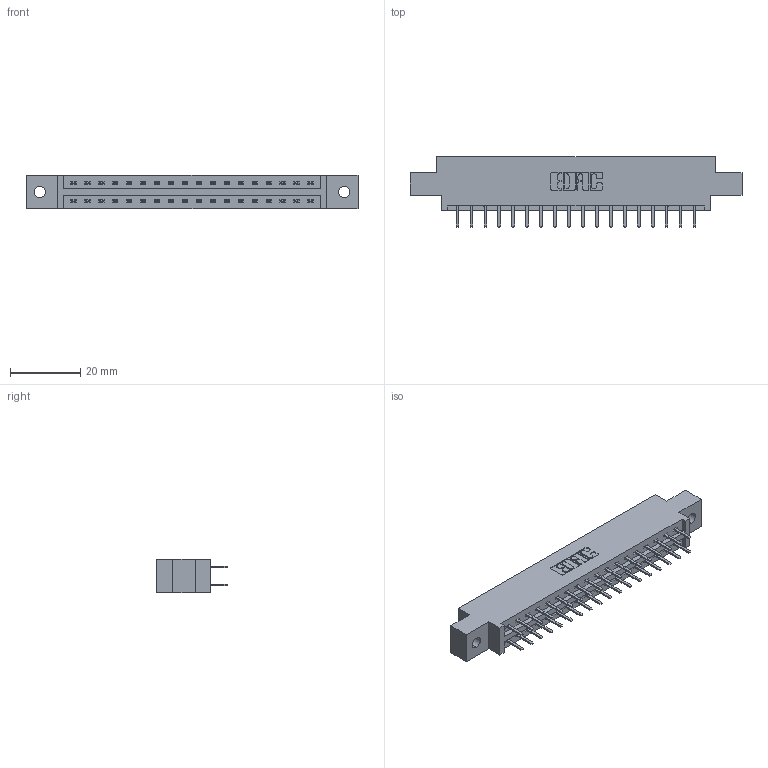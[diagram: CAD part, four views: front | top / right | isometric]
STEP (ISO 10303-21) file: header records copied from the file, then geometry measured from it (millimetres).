
FILE_DESCRIPTION (( 'STEP AP203' ), '1' );
FILE_NAME ('387-036-520-802.STEP', '2019-10-17T18:40:45', ( '' ), ( '' ), 'SwSTEP 2.0', 'SolidWorks 2016', '' );
FILE_SCHEMA (( 'CONFIG_CONTROL_DESIGN' ));
Length unit declared in the file: inch
Products named in the file (3): 345-292-001_345-293-120; 387-036-520-802; 337 Part_0.170 Offset - 0.128 Dia
Assembly tree (37 placements, depth 2):
  387-036-520-802
    337 Part_0.170 Offset - 0.128 Dia
    345-292-001_345-293-120  x36
Bounding box: 94.34 x 20.02 x 9.4 mm (x, y, z)
Volume: 9452.4 mm3; surface area: 10242.8 mm2
Topology: 37 solids, 37 shells, 2206 faces, 6407 edges, 4174 vertices
Faces by surface type: plane 1514, cylinder 692
Entity records: 17309 total; most frequent: CARTESIAN_POINT 2950, ORIENTED_EDGE 2874, DIRECTION 2541, EDGE_CURVE 1437, LINE 1305, VECTOR 1305, VERTEX_POINT 954, AXIS2_PLACEMENT_3D 618
